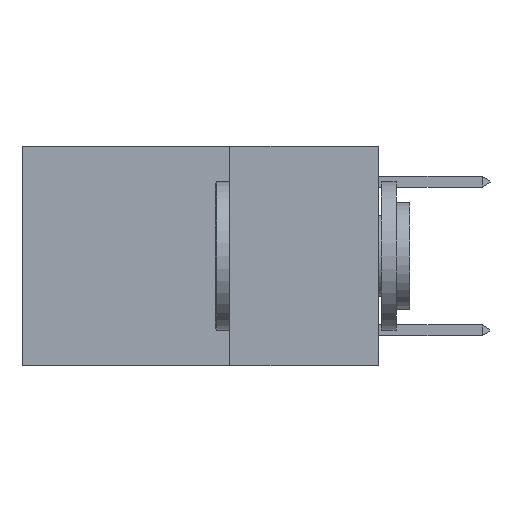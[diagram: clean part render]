
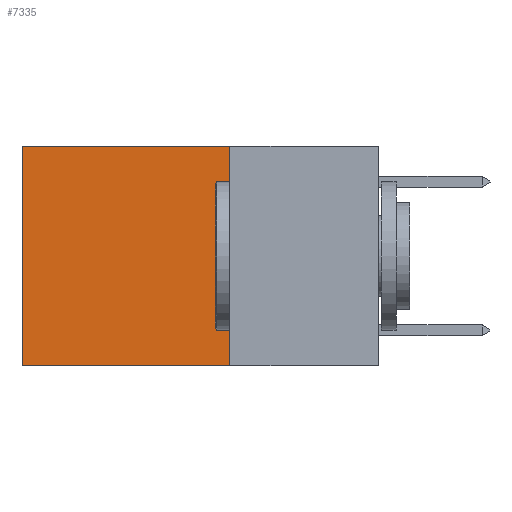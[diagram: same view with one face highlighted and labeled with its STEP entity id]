
A CAD part, left-side view. The second image highlights one B-rep face of the part: STEP entity #7335.
In plain terms, the highlighted planar face has unit normal (-1, 0, 0).
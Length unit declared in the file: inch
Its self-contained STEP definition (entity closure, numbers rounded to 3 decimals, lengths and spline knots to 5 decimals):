
#344 = EDGE_CURVE ( 'NONE', #5157, #7938, #18240, .T. ) ;
#350 = CARTESIAN_POINT ( 'NONE',  ( 0.2625, 0.25, -0.37 ) ) ;
#519 = DIRECTION ( 'NONE',  ( 0., 0., -1. ) ) ;
#955 = VECTOR ( 'NONE', #13827, 39.37008 ) ;
#1127 = DIRECTION ( 'NONE',  ( 0., 1., 0. ) ) ;
#1237 = LINE ( 'NONE', #9680, #9625 ) ;
#2118 = PLANE ( 'NONE',  #11292 ) ;
#2374 = CARTESIAN_POINT ( 'NONE',  ( 0.2625, 0.25, 0. ) ) ;
#2418 = EDGE_CURVE ( 'NONE', #22196, #12449, #13606, .T. ) ;
#3004 = DIRECTION ( 'NONE',  ( 0., 0., -1. ) ) ;
#4599 = CARTESIAN_POINT ( 'NONE',  ( 0.2625, 0.6, 0. ) ) ;
#4709 = ORIENTED_EDGE ( 'NONE', *, *, #17231, .F. ) ;
#4771 = VECTOR ( 'NONE', #3004, 39.37008 ) ;
#5157 = VERTEX_POINT ( 'NONE', #13615 ) ;
#5643 = CARTESIAN_POINT ( 'NONE',  ( 0.2625, 0.25, 0. ) ) ;
#6955 = ORIENTED_EDGE ( 'NONE', *, *, #11266, .T. ) ;
#6960 = EDGE_LOOP ( 'NONE', ( #8621, #4709, #18174, #6955 ) ) ;
#7335 = ADVANCED_FACE ( 'NONE', ( #19821 ), #2118, .F. ) ;
#7938 = VERTEX_POINT ( 'NONE', #9919 ) ;
#8621 = ORIENTED_EDGE ( 'NONE', *, *, #344, .T. ) ;
#9625 = VECTOR ( 'NONE', #1127, 39.37008 ) ;
#9680 = CARTESIAN_POINT ( 'NONE',  ( 0.2625, 0.25, -0.37 ) ) ;
#9743 = LINE ( 'NONE', #16677, #19976 ) ;
#9919 = CARTESIAN_POINT ( 'NONE',  ( 0.2625, 0.6, -0.37 ) ) ;
#11030 = DIRECTION ( 'NONE',  ( 0., 1., 0. ) ) ;
#11104 = DIRECTION ( 'NONE',  ( 1., 0., 0. ) ) ;
#11266 = EDGE_CURVE ( 'NONE', #22196, #5157, #9743, .T. ) ;
#11292 = AXIS2_PLACEMENT_3D ( 'NONE', #5643, #11104, #519 ) ;
#12449 = VERTEX_POINT ( 'NONE', #350 ) ;
#13606 = LINE ( 'NONE', #20618, #955 ) ;
#13615 = CARTESIAN_POINT ( 'NONE',  ( 0.2625, 0.6, 0. ) ) ;
#13827 = DIRECTION ( 'NONE',  ( 0., 0., -1. ) ) ;
#16677 = CARTESIAN_POINT ( 'NONE',  ( 0.2625, 0.25, 0. ) ) ;
#17231 = EDGE_CURVE ( 'NONE', #12449, #7938, #1237, .T. ) ;
#18174 = ORIENTED_EDGE ( 'NONE', *, *, #2418, .F. ) ;
#18240 = LINE ( 'NONE', #4599, #4771 ) ;
#19821 = FACE_OUTER_BOUND ( 'NONE', #6960, .T. ) ;
#19976 = VECTOR ( 'NONE', #11030, 39.37008 ) ;
#20618 = CARTESIAN_POINT ( 'NONE',  ( 0.2625, 0.25, 0. ) ) ;
#22196 = VERTEX_POINT ( 'NONE', #2374 ) ;
